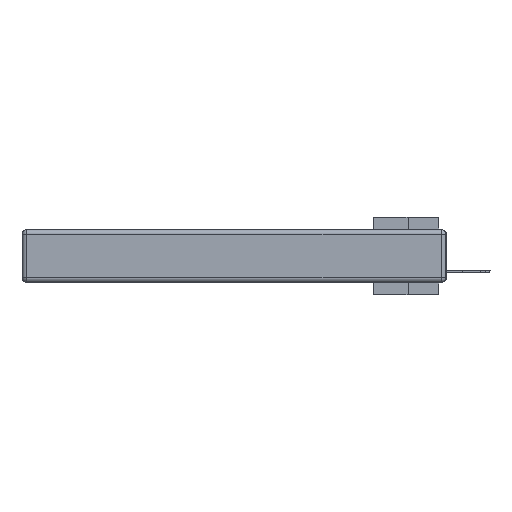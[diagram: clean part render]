
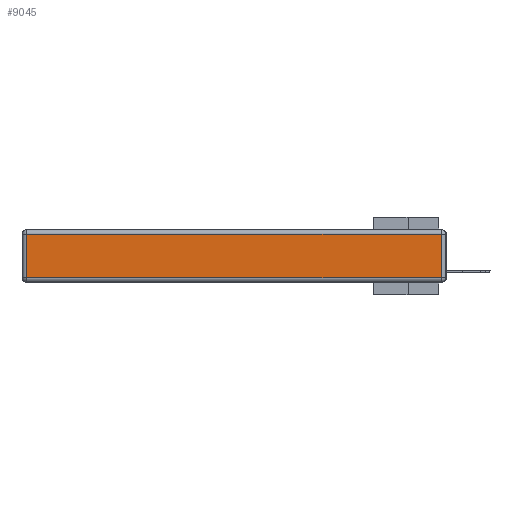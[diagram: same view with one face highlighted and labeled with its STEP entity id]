
A CAD part, left-side view. The second image highlights one B-rep face of the part: STEP entity #9045.
In plain terms, the highlighted planar face has unit normal (-1, 0, 0).
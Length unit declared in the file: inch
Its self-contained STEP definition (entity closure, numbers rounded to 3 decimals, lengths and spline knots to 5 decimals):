
#482 = CARTESIAN_POINT ( 'NONE',  ( 0., 0.03, -0.343 ) ) ;
#516 = VERTEX_POINT ( 'NONE', #11052 ) ;
#1655 = EDGE_CURVE ( 'NONE', #29546, #15229, #29770, .T. ) ;
#2293 = ORIENTED_EDGE ( 'NONE', *, *, #6006, .T. ) ;
#4214 = EDGE_LOOP ( 'NONE', ( #7627, #16818, #24861, #2293 ) ) ;
#4519 = DIRECTION ( 'NONE',  ( 0., -1., 0. ) ) ;
#4532 = PLANE ( 'NONE',  #4939 ) ;
#4939 = AXIS2_PLACEMENT_3D ( 'NONE', #36189, #7755, #10383 ) ;
#6006 = EDGE_CURVE ( 'NONE', #15229, #25625, #36987, .T. ) ;
#6214 = VECTOR ( 'NONE', #32975, 39.37008 ) ;
#7627 = ORIENTED_EDGE ( 'NONE', *, *, #12336, .T. ) ;
#7755 = DIRECTION ( 'NONE',  ( -1., 0., 0. ) ) ;
#8166 = DIRECTION ( 'NONE',  ( 0., 0., -1. ) ) ;
#8804 = LINE ( 'NONE', #482, #17288 ) ;
#9045 = ADVANCED_FACE ( 'NONE', ( #30350 ), #4532, .T. ) ;
#10109 = CARTESIAN_POINT ( 'NONE',  ( 0., 2.72, -0.03 ) ) ;
#10252 = CARTESIAN_POINT ( 'NONE',  ( 0., 0.03, -0.03 ) ) ;
#10383 = DIRECTION ( 'NONE',  ( 0., 0., 1. ) ) ;
#11052 = CARTESIAN_POINT ( 'NONE',  ( 0., 0.03, -0.313 ) ) ;
#11956 = VECTOR ( 'NONE', #8166, 39.37008 ) ;
#12336 = EDGE_CURVE ( 'NONE', #25625, #516, #27128, .T. ) ;
#12824 = CARTESIAN_POINT ( 'NONE',  ( 0., 2.75, -0.03 ) ) ;
#13523 = VECTOR ( 'NONE', #4519, 39.37008 ) ;
#15128 = EDGE_CURVE ( 'NONE', #516, #29546, #8804, .T. ) ;
#15229 = VERTEX_POINT ( 'NONE', #10109 ) ;
#16818 = ORIENTED_EDGE ( 'NONE', *, *, #15128, .T. ) ;
#17288 = VECTOR ( 'NONE', #20299, 39.37008 ) ;
#19233 = CARTESIAN_POINT ( 'NONE',  ( 0., 2.72, -0.313 ) ) ;
#20021 = CARTESIAN_POINT ( 'NONE',  ( 0., 2.72, -0.343 ) ) ;
#20299 = DIRECTION ( 'NONE',  ( 0., 0., 1. ) ) ;
#24861 = ORIENTED_EDGE ( 'NONE', *, *, #1655, .T. ) ;
#25625 = VERTEX_POINT ( 'NONE', #19233 ) ;
#27128 = LINE ( 'NONE', #32977, #13523 ) ;
#29546 = VERTEX_POINT ( 'NONE', #10252 ) ;
#29770 = LINE ( 'NONE', #12824, #6214 ) ;
#30350 = FACE_OUTER_BOUND ( 'NONE', #4214, .T. ) ;
#32975 = DIRECTION ( 'NONE',  ( 0., 1., 0. ) ) ;
#32977 = CARTESIAN_POINT ( 'NONE',  ( 0., 0., -0.313 ) ) ;
#36189 = CARTESIAN_POINT ( 'NONE',  ( 0., 0., -0.343 ) ) ;
#36987 = LINE ( 'NONE', #20021, #11956 ) ;
